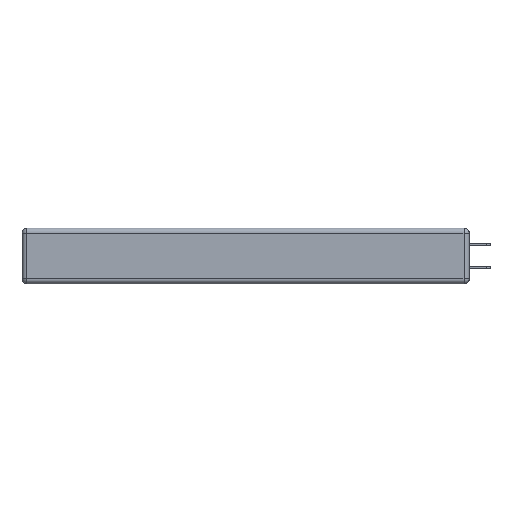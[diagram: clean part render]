
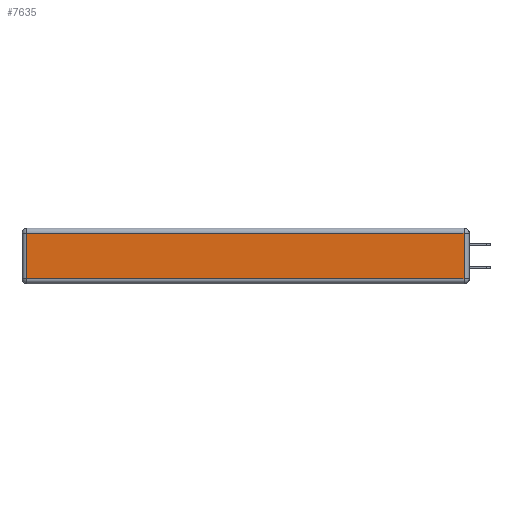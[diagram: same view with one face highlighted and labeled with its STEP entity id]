
A CAD part, left-side view. The second image highlights one B-rep face of the part: STEP entity #7635.
In plain terms, the highlighted planar face has unit normal (-1, 0, 0).
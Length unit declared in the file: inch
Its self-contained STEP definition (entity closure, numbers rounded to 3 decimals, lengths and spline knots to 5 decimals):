
#28 = CARTESIAN_POINT ( 'NONE',  ( 0., 2.72, -0.313 ) ) ;
#230 = LINE ( 'NONE', #2931, #3344 ) ;
#339 = VECTOR ( 'NONE', #8276, 39.37008 ) ;
#551 = AXIS2_PLACEMENT_3D ( 'NONE', #1488, #2542, #3710 ) ;
#826 = EDGE_CURVE ( 'NONE', #3317, #12762, #11091, .T. ) ;
#846 = DIRECTION ( 'NONE',  ( 0., 1., 0. ) ) ;
#935 = CARTESIAN_POINT ( 'NONE',  ( 0., 0.03, -0.343 ) ) ;
#1488 = CARTESIAN_POINT ( 'NONE',  ( 0., 0., -0.343 ) ) ;
#1674 = FACE_OUTER_BOUND ( 'NONE', #7347, .T. ) ;
#1744 = CARTESIAN_POINT ( 'NONE',  ( 0., 0.03, -0.313 ) ) ;
#2542 = DIRECTION ( 'NONE',  ( -1., 0., 0. ) ) ;
#2931 = CARTESIAN_POINT ( 'NONE',  ( 0., 0., -0.313 ) ) ;
#3151 = ORIENTED_EDGE ( 'NONE', *, *, #4146, .T. ) ;
#3317 = VERTEX_POINT ( 'NONE', #1744 ) ;
#3344 = VECTOR ( 'NONE', #12286, 39.37008 ) ;
#3710 = DIRECTION ( 'NONE',  ( 0., 0., 1. ) ) ;
#3728 = CARTESIAN_POINT ( 'NONE',  ( 0., 2.72, -0.03 ) ) ;
#4146 = EDGE_CURVE ( 'NONE', #8715, #3317, #230, .T. ) ;
#4904 = VECTOR ( 'NONE', #8239, 39.37008 ) ;
#5087 = CARTESIAN_POINT ( 'NONE',  ( 0., 2.72, -0.343 ) ) ;
#5105 = CARTESIAN_POINT ( 'NONE',  ( 0., 2.75, -0.03 ) ) ;
#5871 = PLANE ( 'NONE',  #551 ) ;
#7140 = ORIENTED_EDGE ( 'NONE', *, *, #13008, .T. ) ;
#7347 = EDGE_LOOP ( 'NONE', ( #3151, #9981, #9093, #7140 ) ) ;
#7635 = ADVANCED_FACE ( 'NONE', ( #1674 ), #5871, .T. ) ;
#8239 = DIRECTION ( 'NONE',  ( 0., 0., 1. ) ) ;
#8276 = DIRECTION ( 'NONE',  ( 0., 0., -1. ) ) ;
#8715 = VERTEX_POINT ( 'NONE', #28 ) ;
#9093 = ORIENTED_EDGE ( 'NONE', *, *, #10110, .T. ) ;
#9981 = ORIENTED_EDGE ( 'NONE', *, *, #826, .T. ) ;
#10110 = EDGE_CURVE ( 'NONE', #12762, #12761, #11037, .T. ) ;
#11037 = LINE ( 'NONE', #5105, #12844 ) ;
#11091 = LINE ( 'NONE', #935, #4904 ) ;
#12144 = CARTESIAN_POINT ( 'NONE',  ( 0., 0.03, -0.03 ) ) ;
#12286 = DIRECTION ( 'NONE',  ( 0., -1., 0. ) ) ;
#12761 = VERTEX_POINT ( 'NONE', #3728 ) ;
#12762 = VERTEX_POINT ( 'NONE', #12144 ) ;
#12844 = VECTOR ( 'NONE', #846, 39.37008 ) ;
#13008 = EDGE_CURVE ( 'NONE', #12761, #8715, #13255, .T. ) ;
#13255 = LINE ( 'NONE', #5087, #339 ) ;
